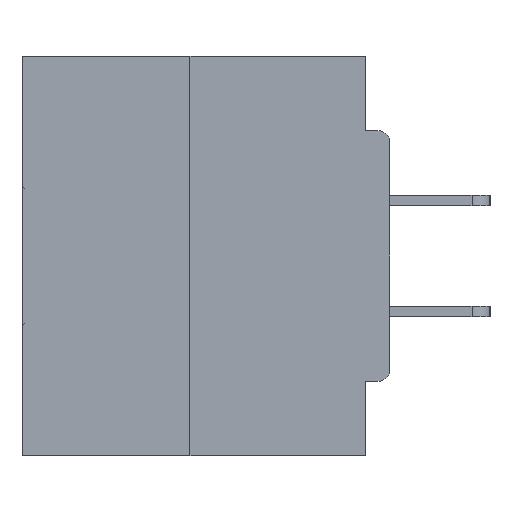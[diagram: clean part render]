
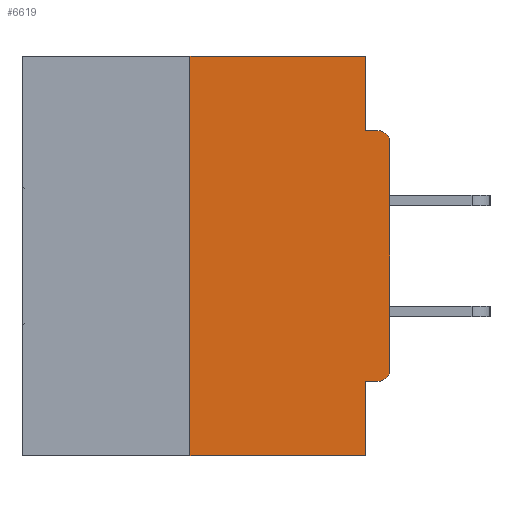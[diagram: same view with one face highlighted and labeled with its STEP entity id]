
A CAD part, left-side view. The second image highlights one B-rep face of the part: STEP entity #6619.
In plain terms, the highlighted planar face has unit normal (-1, 0, 0).
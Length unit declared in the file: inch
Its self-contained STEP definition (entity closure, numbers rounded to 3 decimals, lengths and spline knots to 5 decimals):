
#242 = EDGE_CURVE ( 'NONE', #5189, #31433, #2504, .T. ) ;
#1403 = VECTOR ( 'NONE', #1507, 39.37008 ) ;
#1507 = DIRECTION ( 'NONE',  ( 0., 0., -1. ) ) ;
#1906 = CARTESIAN_POINT ( 'NONE',  ( 0., 0., -0.3915 ) ) ;
#2504 = CIRCLE ( 'NONE', #39983, 0.015 ) ;
#3335 = EDGE_CURVE ( 'NONE', #13039, #20263, #16683, .T. ) ;
#3504 = LINE ( 'NONE', #19824, #20571 ) ;
#3694 = DIRECTION ( 'NONE',  ( 0., -1., 0. ) ) ;
#4278 = PLANE ( 'NONE',  #16370 ) ;
#4296 = ORIENTED_EDGE ( 'NONE', *, *, #34551, .F. ) ;
#4740 = CARTESIAN_POINT ( 'NONE',  ( 0., 0.031, -0.5 ) ) ;
#5189 = VERTEX_POINT ( 'NONE', #17067 ) ;
#5360 = DIRECTION ( 'NONE',  ( 0., 1., 0. ) ) ;
#5838 = DIRECTION ( 'NONE',  ( 0., 0., -1. ) ) ;
#5845 = LINE ( 'NONE', #15303, #30520 ) ;
#6619 = ADVANCED_FACE ( 'NONE', ( #25109 ), #4278, .F. ) ;
#6694 = VERTEX_POINT ( 'NONE', #1906 ) ;
#7195 = EDGE_LOOP ( 'NONE', ( #10715, #35349, #14980, #18045, #20904, #29077, #15800, #10481, #16234, #4296 ) ) ;
#8852 = VERTEX_POINT ( 'NONE', #40122 ) ;
#9797 = DIRECTION ( 'NONE',  ( 0., -1., 0. ) ) ;
#9906 = CARTESIAN_POINT ( 'NONE',  ( 0., 0.031, -0.0935 ) ) ;
#10092 = VERTEX_POINT ( 'NONE', #4740 ) ;
#10367 = CARTESIAN_POINT ( 'NONE',  ( 0., 0.031, -0.5 ) ) ;
#10481 = ORIENTED_EDGE ( 'NONE', *, *, #242, .T. ) ;
#10591 = VERTEX_POINT ( 'NONE', #12119 ) ;
#10715 = ORIENTED_EDGE ( 'NONE', *, *, #26470, .F. ) ;
#11589 = DIRECTION ( 'NONE',  ( 0., -1., 0. ) ) ;
#12119 = CARTESIAN_POINT ( 'NONE',  ( 0., 0.031, 0. ) ) ;
#13039 = VERTEX_POINT ( 'NONE', #40903 ) ;
#14008 = VECTOR ( 'NONE', #11589, 39.37008 ) ;
#14915 = EDGE_CURVE ( 'NONE', #13039, #10092, #23168, .T. ) ;
#14980 = ORIENTED_EDGE ( 'NONE', *, *, #14915, .T. ) ;
#15201 = VECTOR ( 'NONE', #24287, 39.37008 ) ;
#15303 = CARTESIAN_POINT ( 'NONE',  ( 0., 0., -0.4065 ) ) ;
#15382 = DIRECTION ( 'NONE',  ( -1., 0., 0. ) ) ;
#15706 = VECTOR ( 'NONE', #33039, 39.37008 ) ;
#15800 = ORIENTED_EDGE ( 'NONE', *, *, #23086, .T. ) ;
#16234 = ORIENTED_EDGE ( 'NONE', *, *, #33513, .F. ) ;
#16370 = AXIS2_PLACEMENT_3D ( 'NONE', #26759, #33242, #36526 ) ;
#16597 = EDGE_CURVE ( 'NONE', #27647, #6694, #35170, .T. ) ;
#16683 = LINE ( 'NONE', #39859, #21219 ) ;
#17067 = CARTESIAN_POINT ( 'NONE',  ( 0., 0., -0.1085 ) ) ;
#17734 = LINE ( 'NONE', #10367, #15706 ) ;
#18045 = ORIENTED_EDGE ( 'NONE', *, *, #30970, .F. ) ;
#18523 = CARTESIAN_POINT ( 'NONE',  ( 0., 0.25, 0. ) ) ;
#18535 = DIRECTION ( 'NONE',  ( 0., 0., 1. ) ) ;
#19317 = CARTESIAN_POINT ( 'NONE',  ( 0., 0.015, -0.1085 ) ) ;
#19824 = CARTESIAN_POINT ( 'NONE',  ( 0., 0.46, 0. ) ) ;
#20164 = CARTESIAN_POINT ( 'NONE',  ( 0., 0.015, -0.0935 ) ) ;
#20263 = VERTEX_POINT ( 'NONE', #18523 ) ;
#20298 = VERTEX_POINT ( 'NONE', #9906 ) ;
#20442 = CARTESIAN_POINT ( 'NONE',  ( 0., 0.031, 0. ) ) ;
#20571 = VECTOR ( 'NONE', #3694, 39.37008 ) ;
#20904 = ORIENTED_EDGE ( 'NONE', *, *, #35073, .F. ) ;
#21219 = VECTOR ( 'NONE', #18535, 39.37008 ) ;
#23086 = EDGE_CURVE ( 'NONE', #6694, #5189, #34372, .T. ) ;
#23168 = LINE ( 'NONE', #35173, #34323 ) ;
#23456 = CARTESIAN_POINT ( 'NONE',  ( 0., 0.015, -0.4065 ) ) ;
#24287 = DIRECTION ( 'NONE',  ( 0., 0., 1. ) ) ;
#24680 = CARTESIAN_POINT ( 'NONE',  ( 0., 0.015, -0.3915 ) ) ;
#25109 = FACE_OUTER_BOUND ( 'NONE', #7195, .T. ) ;
#26092 = DIRECTION ( 'NONE',  ( -1., 0., 0. ) ) ;
#26470 = EDGE_CURVE ( 'NONE', #20263, #10591, #3504, .T. ) ;
#26759 = CARTESIAN_POINT ( 'NONE',  ( 0., 0.46, 0. ) ) ;
#27639 = CARTESIAN_POINT ( 'NONE',  ( 0., 0., -0.0935 ) ) ;
#27647 = VERTEX_POINT ( 'NONE', #23456 ) ;
#29077 = ORIENTED_EDGE ( 'NONE', *, *, #16597, .T. ) ;
#30520 = VECTOR ( 'NONE', #5360, 39.37008 ) ;
#30970 = EDGE_CURVE ( 'NONE', #8852, #10092, #17734, .T. ) ;
#31433 = VERTEX_POINT ( 'NONE', #20164 ) ;
#32032 = DIRECTION ( 'NONE',  ( 0., 0., -1. ) ) ;
#32548 = AXIS2_PLACEMENT_3D ( 'NONE', #24680, #15382, #5838 ) ;
#33039 = DIRECTION ( 'NONE',  ( 0., 0., -1. ) ) ;
#33242 = DIRECTION ( 'NONE',  ( 1., 0., 0. ) ) ;
#33513 = EDGE_CURVE ( 'NONE', #20298, #31433, #33658, .T. ) ;
#33658 = LINE ( 'NONE', #27639, #14008 ) ;
#33754 = CARTESIAN_POINT ( 'NONE',  ( 0., 0., 0. ) ) ;
#34323 = VECTOR ( 'NONE', #9797, 39.37008 ) ;
#34372 = LINE ( 'NONE', #33754, #15201 ) ;
#34551 = EDGE_CURVE ( 'NONE', #10591, #20298, #40662, .T. ) ;
#35073 = EDGE_CURVE ( 'NONE', #27647, #8852, #5845, .T. ) ;
#35170 = CIRCLE ( 'NONE', #32548, 0.015 ) ;
#35173 = CARTESIAN_POINT ( 'NONE',  ( 0., 0.46, -0.5 ) ) ;
#35349 = ORIENTED_EDGE ( 'NONE', *, *, #3335, .F. ) ;
#36526 = DIRECTION ( 'NONE',  ( 0., 0., -1. ) ) ;
#39859 = CARTESIAN_POINT ( 'NONE',  ( 0., 0.25, 0. ) ) ;
#39983 = AXIS2_PLACEMENT_3D ( 'NONE', #19317, #26092, #32032 ) ;
#40122 = CARTESIAN_POINT ( 'NONE',  ( 0., 0.031, -0.4065 ) ) ;
#40662 = LINE ( 'NONE', #20442, #1403 ) ;
#40903 = CARTESIAN_POINT ( 'NONE',  ( 0., 0.25, -0.5 ) ) ;
